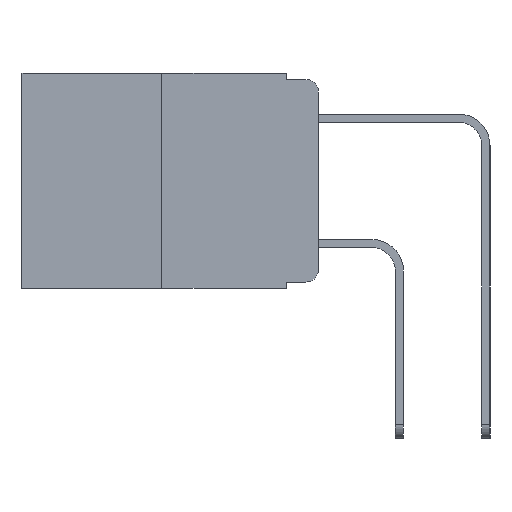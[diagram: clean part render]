
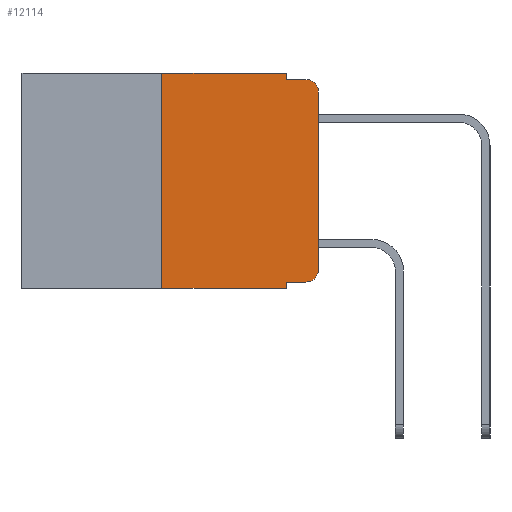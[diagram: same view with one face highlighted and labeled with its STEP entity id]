
A CAD part, left-side view. The second image highlights one B-rep face of the part: STEP entity #12114.
In plain terms, the highlighted planar face has unit normal (-1, 0, 0).
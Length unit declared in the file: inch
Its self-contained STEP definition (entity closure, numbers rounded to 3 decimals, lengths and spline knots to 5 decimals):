
#381 = EDGE_CURVE ( 'NONE', #7633, #10980, #3394, .T. ) ;
#460 = CARTESIAN_POINT ( 'NONE',  ( 0., 0.02, -0.01 ) ) ;
#486 = EDGE_CURVE ( 'NONE', #791, #2720, #9199, .T. ) ;
#547 = VERTEX_POINT ( 'NONE', #1487 ) ;
#591 = EDGE_CURVE ( 'NONE', #8623, #7633, #3215, .T. ) ;
#791 = VERTEX_POINT ( 'NONE', #5080 ) ;
#1309 = ORIENTED_EDGE ( 'NONE', *, *, #6718, .F. ) ;
#1487 = CARTESIAN_POINT ( 'NONE',  ( 0., 0.25, -0.343 ) ) ;
#1631 = ORIENTED_EDGE ( 'NONE', *, *, #10361, .T. ) ;
#1657 = EDGE_CURVE ( 'NONE', #9968, #5192, #9767, .T. ) ;
#1832 = VECTOR ( 'NONE', #2830, 39.37008 ) ;
#2137 = DIRECTION ( 'NONE',  ( -1., 0., 0. ) ) ;
#2141 = DIRECTION ( 'NONE',  ( 0., 0., 1. ) ) ;
#2234 = DIRECTION ( 'NONE',  ( 0., -1., 0. ) ) ;
#2444 = FACE_OUTER_BOUND ( 'NONE', #4820, .T. ) ;
#2570 = ORIENTED_EDGE ( 'NONE', *, *, #10142, .T. ) ;
#2720 = VERTEX_POINT ( 'NONE', #3608 ) ;
#2830 = DIRECTION ( 'NONE',  ( 0., 0., -1. ) ) ;
#3115 = VECTOR ( 'NONE', #3901, 39.37008 ) ;
#3215 = LINE ( 'NONE', #10135, #8611 ) ;
#3360 = CARTESIAN_POINT ( 'NONE',  ( 0., 0.051, -0.01 ) ) ;
#3394 = CIRCLE ( 'NONE', #8891, 0.02 ) ;
#3437 = DIRECTION ( 'NONE',  ( 0., -1., 0. ) ) ;
#3564 = DIRECTION ( 'NONE',  ( 1., 0., 0. ) ) ;
#3608 = CARTESIAN_POINT ( 'NONE',  ( 0., 0.051, -0.01 ) ) ;
#3827 = CIRCLE ( 'NONE', #11713, 0.02 ) ;
#3901 = DIRECTION ( 'NONE',  ( 0., 0., 1. ) ) ;
#4309 = DIRECTION ( 'NONE',  ( 0., 0., -1. ) ) ;
#4458 = VECTOR ( 'NONE', #2234, 39.37008 ) ;
#4578 = ORIENTED_EDGE ( 'NONE', *, *, #1657, .T. ) ;
#4751 = EDGE_CURVE ( 'NONE', #7459, #791, #7532, .T. ) ;
#4820 = EDGE_LOOP ( 'NONE', ( #10017, #12438, #10329, #10903, #6243, #1309, #1631, #9302, #4578, #2570 ) ) ;
#4991 = VECTOR ( 'NONE', #7923, 39.37008 ) ;
#5080 = CARTESIAN_POINT ( 'NONE',  ( 0., 0.051, 0. ) ) ;
#5192 = VERTEX_POINT ( 'NONE', #7039 ) ;
#5493 = CARTESIAN_POINT ( 'NONE',  ( 0., 0.473, 0. ) ) ;
#6012 = CARTESIAN_POINT ( 'NONE',  ( 0., 0.02, -0.03 ) ) ;
#6243 = ORIENTED_EDGE ( 'NONE', *, *, #4751, .F. ) ;
#6270 = VECTOR ( 'NONE', #3437, 39.37008 ) ;
#6353 = CARTESIAN_POINT ( 'NONE',  ( 0., 0.051, -0.333 ) ) ;
#6563 = LINE ( 'NONE', #11017, #6270 ) ;
#6646 = CARTESIAN_POINT ( 'NONE',  ( 0., 0.473, 0. ) ) ;
#6718 = EDGE_CURVE ( 'NONE', #547, #7459, #8258, .T. ) ;
#6897 = CARTESIAN_POINT ( 'NONE',  ( 0., 0.051, -0.343 ) ) ;
#7036 = VECTOR ( 'NONE', #9993, 39.37008 ) ;
#7039 = CARTESIAN_POINT ( 'NONE',  ( 0., 0.02, -0.333 ) ) ;
#7274 = CARTESIAN_POINT ( 'NONE',  ( 0., 0., -0.03 ) ) ;
#7459 = VERTEX_POINT ( 'NONE', #10677 ) ;
#7479 = VECTOR ( 'NONE', #7806, 39.37008 ) ;
#7532 = LINE ( 'NONE', #6646, #4991 ) ;
#7633 = VERTEX_POINT ( 'NONE', #7274 ) ;
#7806 = DIRECTION ( 'NONE',  ( 0., 0., -1. ) ) ;
#7919 = VERTEX_POINT ( 'NONE', #6897 ) ;
#7923 = DIRECTION ( 'NONE',  ( 0., -1., 0. ) ) ;
#7946 = CARTESIAN_POINT ( 'NONE',  ( 0., 0.02, -0.313 ) ) ;
#8041 = AXIS2_PLACEMENT_3D ( 'NONE', #5493, #3564, #10200 ) ;
#8258 = LINE ( 'NONE', #12302, #3115 ) ;
#8611 = VECTOR ( 'NONE', #2141, 39.37008 ) ;
#8623 = VERTEX_POINT ( 'NONE', #10768 ) ;
#8718 = CARTESIAN_POINT ( 'NONE',  ( 0., 0.051, 0. ) ) ;
#8863 = DIRECTION ( 'NONE',  ( 0., 0., -1. ) ) ;
#8891 = AXIS2_PLACEMENT_3D ( 'NONE', #6012, #12245, #4309 ) ;
#9199 = LINE ( 'NONE', #11512, #1832 ) ;
#9261 = PLANE ( 'NONE',  #8041 ) ;
#9302 = ORIENTED_EDGE ( 'NONE', *, *, #9398, .F. ) ;
#9398 = EDGE_CURVE ( 'NONE', #9968, #7919, #9926, .T. ) ;
#9487 = LINE ( 'NONE', #3360, #7036 ) ;
#9649 = EDGE_CURVE ( 'NONE', #2720, #10980, #9487, .T. ) ;
#9767 = LINE ( 'NONE', #6353, #4458 ) ;
#9926 = LINE ( 'NONE', #8718, #7479 ) ;
#9968 = VERTEX_POINT ( 'NONE', #11366 ) ;
#9993 = DIRECTION ( 'NONE',  ( 0., -1., 0. ) ) ;
#10017 = ORIENTED_EDGE ( 'NONE', *, *, #591, .T. ) ;
#10135 = CARTESIAN_POINT ( 'NONE',  ( 0., 0., 0. ) ) ;
#10142 = EDGE_CURVE ( 'NONE', #5192, #8623, #3827, .T. ) ;
#10200 = DIRECTION ( 'NONE',  ( 0., 0., -1. ) ) ;
#10329 = ORIENTED_EDGE ( 'NONE', *, *, #9649, .F. ) ;
#10361 = EDGE_CURVE ( 'NONE', #547, #7919, #6563, .T. ) ;
#10677 = CARTESIAN_POINT ( 'NONE',  ( 0., 0.25, 0. ) ) ;
#10768 = CARTESIAN_POINT ( 'NONE',  ( 0., 0., -0.313 ) ) ;
#10903 = ORIENTED_EDGE ( 'NONE', *, *, #486, .F. ) ;
#10980 = VERTEX_POINT ( 'NONE', #460 ) ;
#11017 = CARTESIAN_POINT ( 'NONE',  ( 0., 0.473, -0.343 ) ) ;
#11366 = CARTESIAN_POINT ( 'NONE',  ( 0., 0.051, -0.333 ) ) ;
#11512 = CARTESIAN_POINT ( 'NONE',  ( 0., 0.051, 0. ) ) ;
#11713 = AXIS2_PLACEMENT_3D ( 'NONE', #7946, #2137, #8863 ) ;
#12114 = ADVANCED_FACE ( 'NONE', ( #2444 ), #9261, .F. ) ;
#12245 = DIRECTION ( 'NONE',  ( -1., 0., 0. ) ) ;
#12302 = CARTESIAN_POINT ( 'NONE',  ( 0., 0.25, 0. ) ) ;
#12438 = ORIENTED_EDGE ( 'NONE', *, *, #381, .T. ) ;
